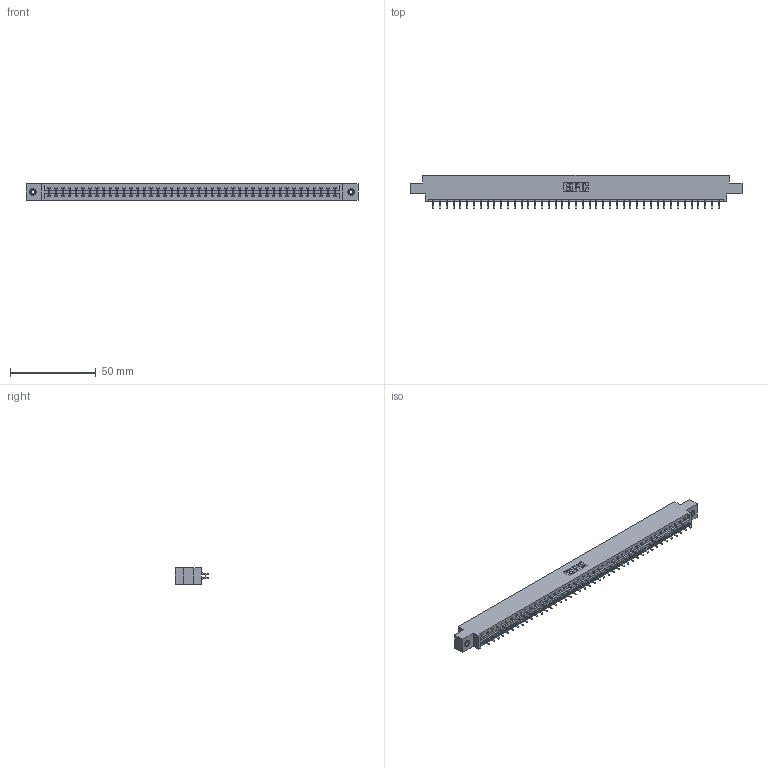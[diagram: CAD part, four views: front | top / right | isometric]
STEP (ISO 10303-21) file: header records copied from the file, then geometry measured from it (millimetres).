
FILE_DESCRIPTION (( 'STEP AP203' ), '1' );
FILE_NAME ('387-086-556-808.STEP', '2019-10-23T04:20:37', ( '' ), ( '' ), 'SwSTEP 2.0', 'SolidWorks 2016', '' );
FILE_SCHEMA (( 'CONFIG_CONTROL_DESIGN' ));
Length unit declared in the file: inch
Products named in the file (4): 387-086-556-808; 337 Part_0.170 Offset - 0.156 Dia-TI; 345-292-001_556 Tail; 345-250-001_345-250-003-102
Assembly tree (89 placements, depth 2):
  387-086-556-808
    337 Part_0.170 Offset - 0.156 Dia-TI
    345-292-001_556 Tail  x86
    345-250-001_345-250-003-102  x2
Bounding box: 193.4 x 19.57 x 9.4 mm (x, y, z)
Volume: 20267.4 mm3; surface area: 22963.1 mm2
Topology: 89 solids, 89 shells, 5338 faces, 15853 edges, 10446 vertices
Faces by surface type: plane 3718, cylinder 1604, cone 12, torus 4
Entity records: 34748 total; most frequent: CARTESIAN_POINT 5849, ORIENTED_EDGE 5766, DIRECTION 4993, EDGE_CURVE 2883, VECTOR 2727, LINE 2727, VERTEX_POINT 1916, AXIS2_PLACEMENT_3D 1133
